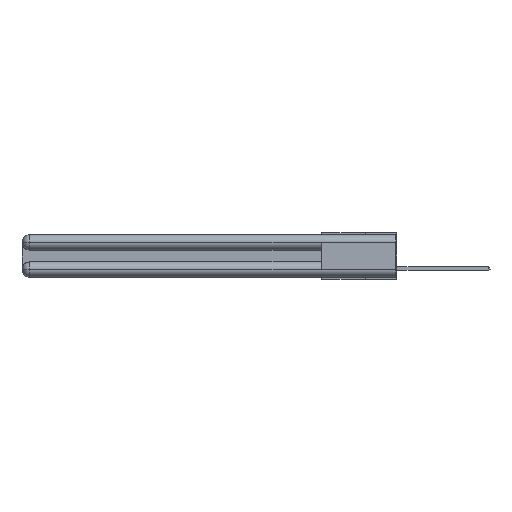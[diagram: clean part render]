
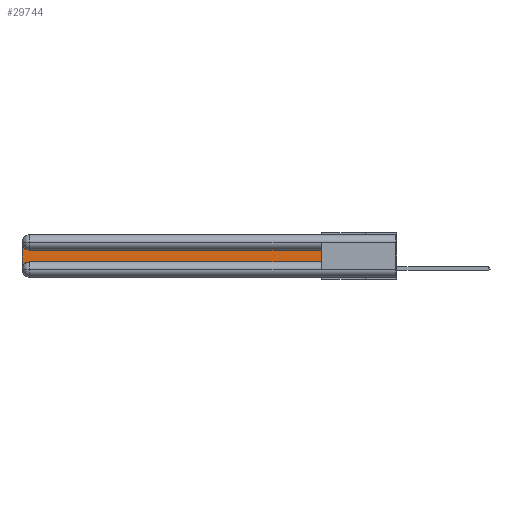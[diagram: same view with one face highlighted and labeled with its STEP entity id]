
A CAD part, left-side view. The second image highlights one B-rep face of the part: STEP entity #29744.
In plain terms, the highlighted planar face has unit normal (-1, 0, 0).
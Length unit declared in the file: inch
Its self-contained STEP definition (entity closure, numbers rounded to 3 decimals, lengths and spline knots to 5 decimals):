
#31 = EDGE_LOOP ( 'NONE', ( #19422, #14204, #1818, #6638, #9917, #15982 ) ) ;
#399 = LINE ( 'NONE', #17501, #30486 ) ;
#1744 = VERTEX_POINT ( 'NONE', #26545 ) ;
#1818 = ORIENTED_EDGE ( 'NONE', *, *, #27021, .T. ) ;
#2591 = DIRECTION ( 'NONE',  ( 1., 0., 0. ) ) ;
#2677 = VERTEX_POINT ( 'NONE', #27520 ) ;
#2917 = EDGE_CURVE ( 'NONE', #2677, #21316, #19091, .T. ) ;
#3097 = DIRECTION ( 'NONE',  ( 0., -1., 0. ) ) ;
#3322 = CARTESIAN_POINT ( 'NONE',  ( 0.075, 0.6, -0.1225 ) ) ;
#4052 = DIRECTION ( 'NONE',  ( 0., 0., -1. ) ) ;
#4408 = LINE ( 'NONE', #12209, #24115 ) ;
#4792 = LINE ( 'NONE', #3322, #16683 ) ;
#5240 = VERTEX_POINT ( 'NONE', #19691 ) ;
#5566 = DIRECTION ( 'NONE',  ( 0., 1., 0. ) ) ;
#6638 = ORIENTED_EDGE ( 'NONE', *, *, #2917, .T. ) ;
#9788 = CARTESIAN_POINT ( 'NONE',  ( 0.075, 3., -0.1225 ) ) ;
#9917 = ORIENTED_EDGE ( 'NONE', *, *, #17360, .T. ) ;
#10080 = CARTESIAN_POINT ( 'NONE',  ( 0.075, 2.94, -0.2175 ) ) ;
#10929 = AXIS2_PLACEMENT_3D ( 'NONE', #11426, #11009, #4052 ) ;
#11009 = DIRECTION ( 'NONE',  ( 1., 0., 0. ) ) ;
#11426 = CARTESIAN_POINT ( 'NONE',  ( 0.075, 2.94, -0.2775 ) ) ;
#12088 = CARTESIAN_POINT ( 'NONE',  ( 0.075, 3., -0.0625 ) ) ;
#12209 = CARTESIAN_POINT ( 'NONE',  ( 0.075, 0.6, -0.2175 ) ) ;
#12419 = DIRECTION ( 'NONE',  ( 0., 0., -1. ) ) ;
#12660 = CARTESIAN_POINT ( 'NONE',  ( 0.075, 0.6, -0.2175 ) ) ;
#13098 = CARTESIAN_POINT ( 'NONE',  ( 0.075, 2.94, -0.1225 ) ) ;
#14204 = ORIENTED_EDGE ( 'NONE', *, *, #18290, .T. ) ;
#14590 = EDGE_CURVE ( 'NONE', #1744, #5240, #4408, .T. ) ;
#14803 = DIRECTION ( 'NONE',  ( 0., 0., -1. ) ) ;
#14846 = VERTEX_POINT ( 'NONE', #13098 ) ;
#15982 = ORIENTED_EDGE ( 'NONE', *, *, #14590, .T. ) ;
#16683 = VECTOR ( 'NONE', #5566, 39.37008 ) ;
#16964 = CARTESIAN_POINT ( 'NONE',  ( 0.075, 2.94, -0.0625 ) ) ;
#17021 = AXIS2_PLACEMENT_3D ( 'NONE', #16964, #29016, #14803 ) ;
#17360 = EDGE_CURVE ( 'NONE', #21316, #1744, #19395, .T. ) ;
#17501 = CARTESIAN_POINT ( 'NONE',  ( 0.075, 3., -0.2175 ) ) ;
#18290 = EDGE_CURVE ( 'NONE', #14846, #20321, #21926, .T. ) ;
#19091 = CIRCLE ( 'NONE', #10929, 0.06 ) ;
#19395 = LINE ( 'NONE', #12660, #21615 ) ;
#19422 = ORIENTED_EDGE ( 'NONE', *, *, #27719, .T. ) ;
#19691 = CARTESIAN_POINT ( 'NONE',  ( 0.075, 0.6, -0.1225 ) ) ;
#20321 = VERTEX_POINT ( 'NONE', #12088 ) ;
#21316 = VERTEX_POINT ( 'NONE', #10080 ) ;
#21615 = VECTOR ( 'NONE', #3097, 39.37008 ) ;
#21926 = CIRCLE ( 'NONE', #17021, 0.06 ) ;
#24115 = VECTOR ( 'NONE', #28877, 39.37008 ) ;
#25961 = PLANE ( 'NONE',  #30355 ) ;
#25983 = FACE_OUTER_BOUND ( 'NONE', #31, .T. ) ;
#26402 = DIRECTION ( 'NONE',  ( 0., 0., -1. ) ) ;
#26545 = CARTESIAN_POINT ( 'NONE',  ( 0.075, 0.6, -0.2175 ) ) ;
#27021 = EDGE_CURVE ( 'NONE', #20321, #2677, #399, .T. ) ;
#27520 = CARTESIAN_POINT ( 'NONE',  ( 0.075, 3., -0.2775 ) ) ;
#27719 = EDGE_CURVE ( 'NONE', #5240, #14846, #4792, .T. ) ;
#28877 = DIRECTION ( 'NONE',  ( 0., 0., 1. ) ) ;
#29016 = DIRECTION ( 'NONE',  ( 1., 0., 0. ) ) ;
#29744 = ADVANCED_FACE ( 'NONE', ( #25983 ), #25961, .F. ) ;
#30355 = AXIS2_PLACEMENT_3D ( 'NONE', #9788, #2591, #26402 ) ;
#30486 = VECTOR ( 'NONE', #12419, 39.37008 ) ;
